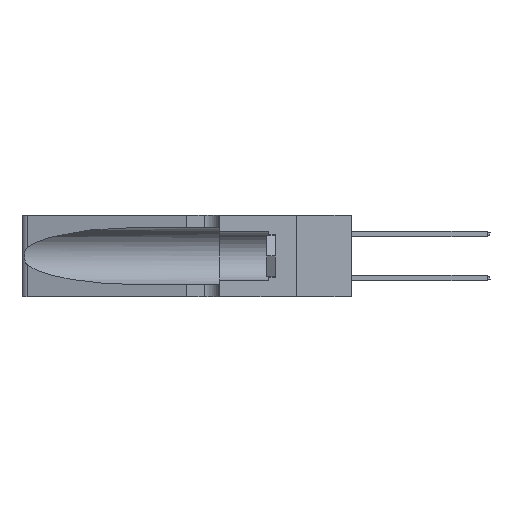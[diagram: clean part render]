
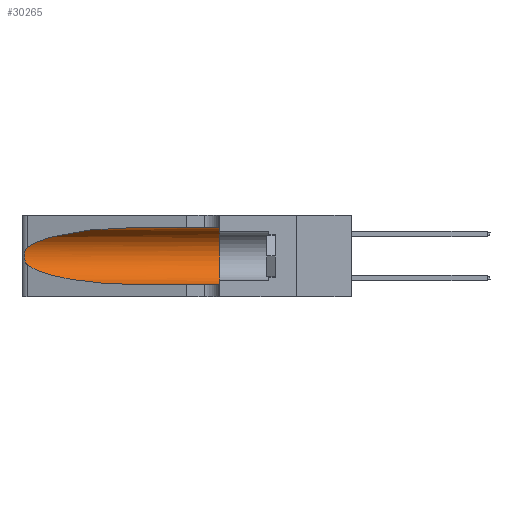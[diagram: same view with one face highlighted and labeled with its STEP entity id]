
A CAD part, left-side view. The second image highlights one B-rep face of the part: STEP entity #30265.
In plain terms, the highlighted cylindrical face has radius 3.308 mm (diameter 6.617 mm), a partial arc.
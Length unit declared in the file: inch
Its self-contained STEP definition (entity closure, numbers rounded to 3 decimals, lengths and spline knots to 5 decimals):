
#1896 = CARTESIAN_POINT ( 'NONE',  ( 0.1305, 1.61858, 0.31525 ) ) ;
#1946 = VECTOR ( 'NONE', #24128, 39.37008 ) ;
#3057 = CARTESIAN_POINT ( 'NONE',  ( 0.25639, 1.23186, 0.15144 ) ) ;
#3097 = VECTOR ( 'NONE', #6375, 39.37008 ) ;
#3166 = B_SPLINE_CURVE_WITH_KNOTS ( 'NONE', 3,
 ( #21929, #25127, #9421, #31435, #12584, #34598, #15778, #37757, #18925, #40918, #22067, #3057, #25265, #6365 ),
 .UNSPECIFIED., .F., .F.,
 ( 4, 2, 2, 2, 2, 2, 4 ),
 ( 0., 0.00027, 0.00053, 0.00107, 0.0016, 0.00187, 0.00214 ),
 .UNSPECIFIED. ) ;
#3912 = VERTEX_POINT ( 'NONE', #25592 ) ;
#3917 = VERTEX_POINT ( 'NONE', #22398 ) ;
#5647 = DIRECTION ( 'NONE',  ( 0., 0., -1. ) ) ;
#5749 = DIRECTION ( 'NONE',  ( 0., 1., 0. ) ) ;
#6275 = VERTEX_POINT ( 'NONE', #11393 ) ;
#6365 = CARTESIAN_POINT ( 'NONE',  ( 0.25487, 1.22718, 0.14631 ) ) ;
#6375 = DIRECTION ( 'NONE',  ( 0., -1., 0. ) ) ;
#7783 = CARTESIAN_POINT ( 'NONE',  ( 0.18966, 0.96281, 0.31525 ) ) ;
#8169 = EDGE_LOOP ( 'NONE', ( #22417, #24939, #12429, #15524, #32658, #31450 ) ) ;
#8780 = CARTESIAN_POINT ( 'NONE',  ( 0.25487, 1.22718, 0.14631 ) ) ;
#9303 = CARTESIAN_POINT ( 'NONE',  ( 0.1305, 0.35, 0.05475 ) ) ;
#9421 = CARTESIAN_POINT ( 'NONE',  ( 0.25639, 1.23184, 0.21858 ) ) ;
#9894 = EDGE_CURVE ( 'NONE', #35482, #35900, #34481, .T. ) ;
#11393 = CARTESIAN_POINT ( 'NONE',  ( 0.1305, 0.72297, 0.31525 ) ) ;
#11714 = AXIS2_PLACEMENT_3D ( 'NONE', #24665, #5749, #27833 ) ;
#12330 = EDGE_CURVE ( 'NONE', #3912, #35900, #36747, .T. ) ;
#12429 = ORIENTED_EDGE ( 'NONE', *, *, #29551, .T. ) ;
#12584 = CARTESIAN_POINT ( 'NONE',  ( 0.25854, 1.2359, 0.20912 ) ) ;
#13731 = EDGE_CURVE ( 'NONE', #6275, #35482, #17951, .T. ) ;
#14122 = CARTESIAN_POINT ( 'NONE',  ( 0.25487, 1.22718, 0.22369 ) ) ;
#15152 = CARTESIAN_POINT ( 'NONE',  ( 0.1305, 0.72297, 0.05475 ) ) ;
#15524 = ORIENTED_EDGE ( 'NONE', *, *, #12330, .T. ) ;
#15778 = CARTESIAN_POINT ( 'NONE',  ( 0.26075, 1.23896, 0.19203 ) ) ;
#16689 = AXIS2_PLACEMENT_3D ( 'NONE', #40229, #24577, #5647 ) ;
#17951 = LINE ( 'NONE', #1896, #1946 ) ;
#18925 = CARTESIAN_POINT ( 'NONE',  ( 0.26017, 1.23833, 0.17102 ) ) ;
#19050 = VERTEX_POINT ( 'NONE', #26346 ) ;
#20212 = CARTESIAN_POINT ( 'NONE',  ( 0.1305, 0.35, 0.31525 ) ) ;
#20410 = EDGE_CURVE ( 'NONE', #19050, #3917, #3166, .T. ) ;
#21929 = CARTESIAN_POINT ( 'NONE',  ( 0.25487, 1.22718, 0.22369 ) ) ;
#22067 = CARTESIAN_POINT ( 'NONE',  ( 0.25789, 1.23486, 0.15765 ) ) ;
#22398 = CARTESIAN_POINT ( 'NONE',  ( 0.25487, 1.22718, 0.14631 ) ) ;
#22417 = ORIENTED_EDGE ( 'NONE', *, *, #30045, .T. ) ;
#24128 = DIRECTION ( 'NONE',  ( 0., -1., 0. ) ) ;
#24577 = DIRECTION ( 'NONE',  ( 0., -1., 0. ) ) ;
#24665 = CARTESIAN_POINT ( 'NONE',  ( 0.1305, 0.35, 0.185 ) ) ;
#24939 = ORIENTED_EDGE ( 'NONE', *, *, #20410, .T. ) ;
#25127 = CARTESIAN_POINT ( 'NONE',  ( 0.25555, 1.22994, 0.2215 ) ) ;
#25265 = CARTESIAN_POINT ( 'NONE',  ( 0.25555, 1.22993, 0.14849 ) ) ;
#25592 = CARTESIAN_POINT ( 'NONE',  ( 0.1305, 0.72297, 0.05475 ) ) ;
#26346 = CARTESIAN_POINT ( 'NONE',  ( 0.25487, 1.22718, 0.22369 ) ) ;
#26578 =( BOUNDED_CURVE ( )  B_SPLINE_CURVE ( 3, ( #29806, #7783, #32956, #14122 ),
 .UNSPECIFIED., .F., .F. ) 
 B_SPLINE_CURVE_WITH_KNOTS ( ( 4, 4 ),
 ( 1.5708, 2.84003 ),
 .UNSPECIFIED. ) 
 CURVE ( )  GEOMETRIC_REPRESENTATION_ITEM ( )  RATIONAL_B_SPLINE_CURVE ( ( 1., 0.87, 0.87, 1. ) ) 
 REPRESENTATION_ITEM ( '' )  );
#27833 = DIRECTION ( 'NONE',  ( 0., 0., 1. ) ) ;
#28433 = CARTESIAN_POINT ( 'NONE',  ( 0.1305, 1.61858, 0.05475 ) ) ;
#29551 = EDGE_CURVE ( 'NONE', #3917, #3912, #33827, .T. ) ;
#29806 = CARTESIAN_POINT ( 'NONE',  ( 0.1305, 0.72297, 0.31525 ) ) ;
#30045 = EDGE_CURVE ( 'NONE', #6275, #19050, #26578, .T. ) ;
#30265 = ADVANCED_FACE ( 'NONE', ( #31300 ), #30307, .F. ) ;
#30307 = CYLINDRICAL_SURFACE ( 'NONE', #16689, 0.13025 ) ;
#30792 = CARTESIAN_POINT ( 'NONE',  ( 0.2373, 1.15595, 0.08982 ) ) ;
#31300 = FACE_OUTER_BOUND ( 'NONE', #8169, .T. ) ;
#31435 = CARTESIAN_POINT ( 'NONE',  ( 0.25787, 1.23484, 0.2124 ) ) ;
#31450 = ORIENTED_EDGE ( 'NONE', *, *, #13731, .F. ) ;
#32658 = ORIENTED_EDGE ( 'NONE', *, *, #9894, .F. ) ;
#32956 = CARTESIAN_POINT ( 'NONE',  ( 0.2373, 1.15595, 0.28018 ) ) ;
#33827 =( BOUNDED_CURVE ( )  B_SPLINE_CURVE ( 3, ( #8780, #30792, #33943, #15152 ),
 .UNSPECIFIED., .F., .T. ) 
 B_SPLINE_CURVE_WITH_KNOTS ( ( 4, 4 ),
 ( 3.44316, 4.71239 ),
 .UNSPECIFIED. ) 
 CURVE ( )  GEOMETRIC_REPRESENTATION_ITEM ( )  RATIONAL_B_SPLINE_CURVE ( ( 1., 0.87, 0.87, 1. ) ) 
 REPRESENTATION_ITEM ( '' )  );
#33943 = CARTESIAN_POINT ( 'NONE',  ( 0.18966, 0.96281, 0.05475 ) ) ;
#34481 = CIRCLE ( 'NONE', #11714, 0.13025 ) ;
#34598 = CARTESIAN_POINT ( 'NONE',  ( 0.26018, 1.23835, 0.19895 ) ) ;
#35482 = VERTEX_POINT ( 'NONE', #20212 ) ;
#35900 = VERTEX_POINT ( 'NONE', #9303 ) ;
#36747 = LINE ( 'NONE', #28433, #3097 ) ;
#37757 = CARTESIAN_POINT ( 'NONE',  ( 0.26075, 1.23896, 0.178 ) ) ;
#40229 = CARTESIAN_POINT ( 'NONE',  ( 0.1305, 1.61858, 0.185 ) ) ;
#40918 = CARTESIAN_POINT ( 'NONE',  ( 0.25856, 1.23593, 0.16098 ) ) ;
